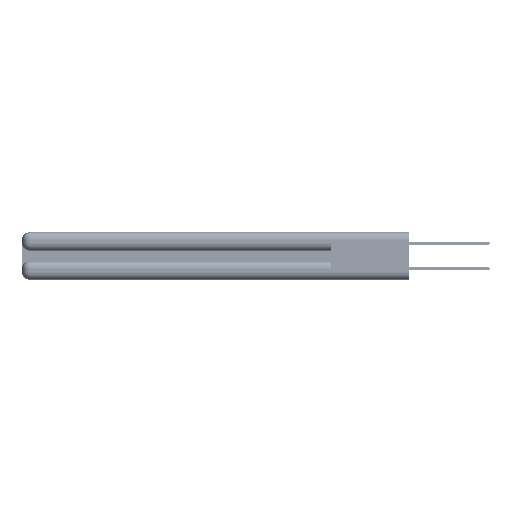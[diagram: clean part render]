
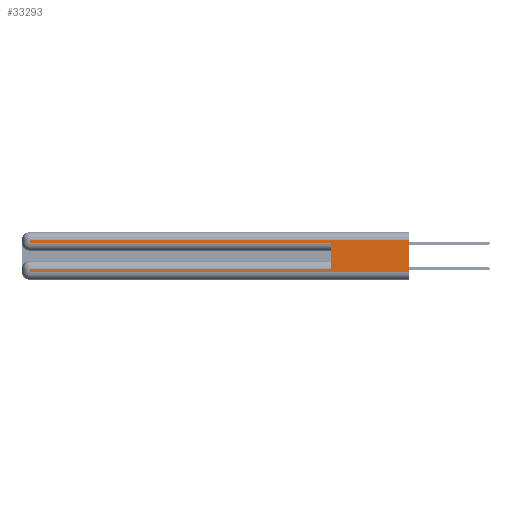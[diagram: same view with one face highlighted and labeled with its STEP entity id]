
A CAD part, left-side view. The second image highlights one B-rep face of the part: STEP entity #33293.
In plain terms, the highlighted planar face has unit normal (-1, 0, 0).
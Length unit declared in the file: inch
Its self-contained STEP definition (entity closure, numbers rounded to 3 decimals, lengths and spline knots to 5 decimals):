
#328 = ORIENTED_EDGE ( 'NONE', *, *, #37271, .F. ) ;
#602 = DIRECTION ( 'NONE',  ( 0., 0., -1. ) ) ;
#743 = CARTESIAN_POINT ( 'NONE',  ( 0., 0., 0.285 ) ) ;
#2374 = CARTESIAN_POINT ( 'NONE',  ( 0., 2.94, 0.31 ) ) ;
#2843 = ORIENTED_EDGE ( 'NONE', *, *, #5191, .T. ) ;
#2849 = CARTESIAN_POINT ( 'NONE',  ( 0., 0., 0.085 ) ) ;
#2942 = CARTESIAN_POINT ( 'NONE',  ( 0., 2.94, 0.085 ) ) ;
#3650 = VERTEX_POINT ( 'NONE', #9985 ) ;
#4491 = EDGE_CURVE ( 'NONE', #12520, #29038, #47456, .T. ) ;
#5191 = EDGE_CURVE ( 'NONE', #49785, #47878, #12978, .T. ) ;
#5424 = VECTOR ( 'NONE', #30754, 39.37008 ) ;
#6039 = DIRECTION ( 'NONE',  ( 0., 1., 0. ) ) ;
#7276 = ORIENTED_EDGE ( 'NONE', *, *, #14458, .T. ) ;
#7741 = DIRECTION ( 'NONE',  ( 0., -1., 0. ) ) ;
#9402 = VECTOR ( 'NONE', #47255, 39.37008 ) ;
#9985 = CARTESIAN_POINT ( 'NONE',  ( 0., 2.94, 0.285 ) ) ;
#11399 = ORIENTED_EDGE ( 'NONE', *, *, #4491, .T. ) ;
#12520 = VERTEX_POINT ( 'NONE', #21518 ) ;
#12948 = CARTESIAN_POINT ( 'NONE',  ( 0., 0., 0.06 ) ) ;
#12978 = LINE ( 'NONE', #43887, #46746 ) ;
#13090 = ORIENTED_EDGE ( 'NONE', *, *, #46451, .T. ) ;
#14458 = EDGE_CURVE ( 'NONE', #24498, #31457, #30068, .T. ) ;
#15136 = EDGE_CURVE ( 'NONE', #3650, #36608, #44482, .T. ) ;
#15578 = CARTESIAN_POINT ( 'NONE',  ( 0., 0., 0.31 ) ) ;
#16036 = CARTESIAN_POINT ( 'NONE',  ( 0., 0.6, 0.285 ) ) ;
#16249 = FACE_OUTER_BOUND ( 'NONE', #42166, .T. ) ;
#16504 = PLANE ( 'NONE',  #24222 ) ;
#17304 = LINE ( 'NONE', #23272, #5424 ) ;
#20331 = CARTESIAN_POINT ( 'NONE',  ( 0., 0.6, 0.145 ) ) ;
#20746 = VECTOR ( 'NONE', #6039, 39.37008 ) ;
#21518 = CARTESIAN_POINT ( 'NONE',  ( 0., 0.6, 0.085 ) ) ;
#21575 = CARTESIAN_POINT ( 'NONE',  ( 0., 0., 0.31 ) ) ;
#23189 = CARTESIAN_POINT ( 'NONE',  ( 0., 2.94, 0.37 ) ) ;
#23272 = CARTESIAN_POINT ( 'NONE',  ( 0., 0., 0.37 ) ) ;
#24222 = AXIS2_PLACEMENT_3D ( 'NONE', #44494, #36228, #602 ) ;
#24498 = VERTEX_POINT ( 'NONE', #15578 ) ;
#25346 = DIRECTION ( 'NONE',  ( 0., -1., 0. ) ) ;
#28648 = VECTOR ( 'NONE', #42536, 39.37008 ) ;
#29038 = VERTEX_POINT ( 'NONE', #2942 ) ;
#30021 = VECTOR ( 'NONE', #25346, 39.37008 ) ;
#30068 = LINE ( 'NONE', #21575, #20746 ) ;
#30754 = DIRECTION ( 'NONE',  ( 0., 0., -1. ) ) ;
#30841 = DIRECTION ( 'NONE',  ( 0., 0., -1. ) ) ;
#31286 = VECTOR ( 'NONE', #30841, 39.37008 ) ;
#31457 = VERTEX_POINT ( 'NONE', #2374 ) ;
#32695 = DIRECTION ( 'NONE',  ( 0., 0., 1. ) ) ;
#33142 = LINE ( 'NONE', #23189, #31286 ) ;
#33293 = ADVANCED_FACE ( 'NONE', ( #16249 ), #16504, .F. ) ;
#34981 = CARTESIAN_POINT ( 'NONE',  ( 0., 2.94, 0.37 ) ) ;
#36228 = DIRECTION ( 'NONE',  ( 1., 0., 0. ) ) ;
#36608 = VERTEX_POINT ( 'NONE', #16036 ) ;
#37271 = EDGE_CURVE ( 'NONE', #12520, #36608, #37926, .T. ) ;
#37703 = EDGE_CURVE ( 'NONE', #24498, #47878, #17304, .T. ) ;
#37926 = LINE ( 'NONE', #20331, #51153 ) ;
#42166 = EDGE_LOOP ( 'NONE', ( #49074, #7276, #44012, #51825, #328, #11399, #13090, #2843 ) ) ;
#42536 = DIRECTION ( 'NONE',  ( 0., 1., 0. ) ) ;
#43120 = LINE ( 'NONE', #34981, #9402 ) ;
#43887 = CARTESIAN_POINT ( 'NONE',  ( 0., 0., 0.06 ) ) ;
#44012 = ORIENTED_EDGE ( 'NONE', *, *, #45712, .T. ) ;
#44482 = LINE ( 'NONE', #743, #30021 ) ;
#44494 = CARTESIAN_POINT ( 'NONE',  ( 0., 0., 0.37 ) ) ;
#45302 = CARTESIAN_POINT ( 'NONE',  ( 0., 2.94, 0.06 ) ) ;
#45712 = EDGE_CURVE ( 'NONE', #31457, #3650, #33142, .T. ) ;
#46451 = EDGE_CURVE ( 'NONE', #29038, #49785, #43120, .T. ) ;
#46746 = VECTOR ( 'NONE', #7741, 39.37008 ) ;
#47255 = DIRECTION ( 'NONE',  ( 0., 0., -1. ) ) ;
#47456 = LINE ( 'NONE', #2849, #28648 ) ;
#47878 = VERTEX_POINT ( 'NONE', #12948 ) ;
#49074 = ORIENTED_EDGE ( 'NONE', *, *, #37703, .F. ) ;
#49785 = VERTEX_POINT ( 'NONE', #45302 ) ;
#51153 = VECTOR ( 'NONE', #32695, 39.37008 ) ;
#51825 = ORIENTED_EDGE ( 'NONE', *, *, #15136, .T. ) ;
